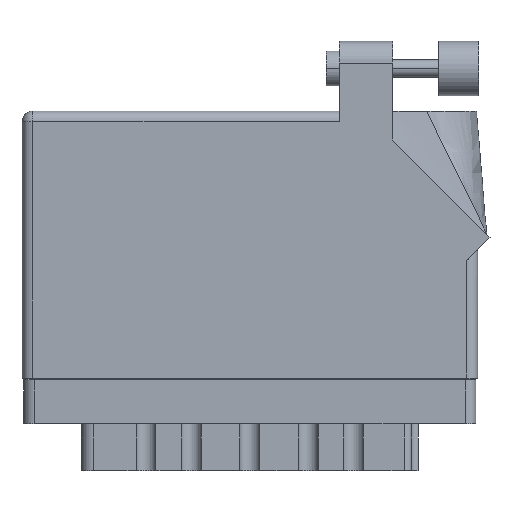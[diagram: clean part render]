
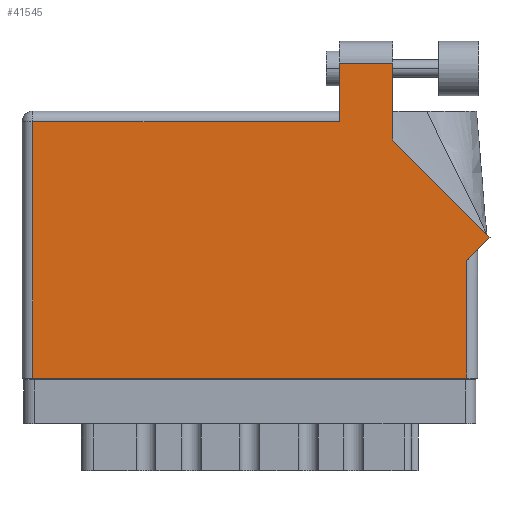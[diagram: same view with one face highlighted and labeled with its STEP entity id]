
A CAD part, front view. The second image highlights one B-rep face of the part: STEP entity #41545.
In plain terms, the highlighted face is planar.
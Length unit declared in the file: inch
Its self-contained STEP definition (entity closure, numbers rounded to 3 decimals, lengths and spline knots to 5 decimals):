
#160 = ORIENTED_EDGE ( 'NONE', *, *, #43689, .T. ) ;
#898 = CARTESIAN_POINT ( 'NONE',  ( 2.126, 1.36442, 0. ) ) ;
#1130 = VECTOR ( 'NONE', #20860, 39.37008 ) ;
#1275 = LINE ( 'NONE', #50636, #2593 ) ;
#1471 = VECTOR ( 'NONE', #4414, 39.37008 ) ;
#2537 = DIRECTION ( 'NONE',  ( -1., 0., 0. ) ) ;
#2593 = VECTOR ( 'NONE', #46176, 39.37008 ) ;
#2642 = CARTESIAN_POINT ( 'NONE',  ( 0., 1.53, 0. ) ) ;
#2730 = VERTEX_POINT ( 'NONE', #9732 ) ;
#2821 = CARTESIAN_POINT ( 'NONE',  ( 1.819, 1.805, 0. ) ) ;
#3860 = VECTOR ( 'NONE', #30760, 39.37008 ) ;
#4414 = DIRECTION ( 'NONE',  ( 0., -1., 0. ) ) ;
#6308 = CARTESIAN_POINT ( 'NONE',  ( 2.55, 0., 0. ) ) ;
#7575 = VERTEX_POINT ( 'NONE', #21977 ) ;
#7707 = VERTEX_POINT ( 'NONE', #2821 ) ;
#8414 = EDGE_CURVE ( 'NONE', #21898, #45044, #1275, .T. ) ;
#8733 = ORIENTED_EDGE ( 'NONE', *, *, #31412, .T. ) ;
#9506 = EDGE_CURVE ( 'NONE', #45044, #24134, #15478, .T. ) ;
#9732 = CARTESIAN_POINT ( 'NONE',  ( 2.126, 1.805, 0. ) ) ;
#10077 = CARTESIAN_POINT ( 'NONE',  ( 0.062, 0., 0. ) ) ;
#10794 = PLANE ( 'NONE',  #29612 ) ;
#10846 = VECTOR ( 'NONE', #25342, 39.37008 ) ;
#10869 = LINE ( 'NONE', #20679, #1130 ) ;
#12183 = ORIENTED_EDGE ( 'NONE', *, *, #40140, .T. ) ;
#12293 = CARTESIAN_POINT ( 'NONE',  ( 2.55, 0.675, 0. ) ) ;
#12740 = VERTEX_POINT ( 'NONE', #34656 ) ;
#13725 = VECTOR ( 'NONE', #2537, 39.37008 ) ;
#13726 = EDGE_CURVE ( 'NONE', #28199, #7575, #24743, .T. ) ;
#13822 = CARTESIAN_POINT ( 'NONE',  ( 2.68271, 0.80771, 0. ) ) ;
#14258 = DIRECTION ( 'NONE',  ( -1., 0., 0. ) ) ;
#14542 = CARTESIAN_POINT ( 'NONE',  ( 2.55, 0.737, 0. ) ) ;
#14940 = ORIENTED_EDGE ( 'NONE', *, *, #13726, .T. ) ;
#15335 = EDGE_CURVE ( 'NONE', #7575, #21898, #50003, .T. ) ;
#15451 = CARTESIAN_POINT ( 'NONE',  ( 2.612, 0.737, 0. ) ) ;
#15478 = LINE ( 'NONE', #14542, #3860 ) ;
#16830 = LINE ( 'NONE', #15451, #38223 ) ;
#16868 = ORIENTED_EDGE ( 'NONE', *, *, #9506, .T. ) ;
#17122 = ORIENTED_EDGE ( 'NONE', *, *, #26634, .T. ) ;
#20679 = CARTESIAN_POINT ( 'NONE',  ( 1.819, 1.53, 0. ) ) ;
#20794 = VECTOR ( 'NONE', #47097, 39.37008 ) ;
#20860 = DIRECTION ( 'NONE',  ( 0., -1., 0. ) ) ;
#21806 = LINE ( 'NONE', #898, #10846 ) ;
#21898 = VERTEX_POINT ( 'NONE', #10077 ) ;
#21977 = CARTESIAN_POINT ( 'NONE',  ( 0.062, 1.468, 0. ) ) ;
#22461 = EDGE_LOOP ( 'NONE', ( #12183, #17122, #52082, #14940, #33768, #53384, #16868, #8733, #160 ) ) ;
#24134 = VERTEX_POINT ( 'NONE', #12293 ) ;
#24701 = CARTESIAN_POINT ( 'NONE',  ( 0.062, 0., 0. ) ) ;
#24743 = LINE ( 'NONE', #44180, #13725 ) ;
#25342 = DIRECTION ( 'NONE',  ( 0., 1., 0. ) ) ;
#25583 = LINE ( 'NONE', #51855, #48249 ) ;
#26634 = EDGE_CURVE ( 'NONE', #2730, #7707, #25583, .T. ) ;
#27177 = DIRECTION ( 'NONE',  ( 0.707, 0.707, 0. ) ) ;
#28199 = VERTEX_POINT ( 'NONE', #52750 ) ;
#29612 = AXIS2_PLACEMENT_3D ( 'NONE', #2642, #31526, #47690 ) ;
#30461 = LINE ( 'NONE', #13822, #20794 ) ;
#30760 = DIRECTION ( 'NONE',  ( 0., 1., 0. ) ) ;
#31412 = EDGE_CURVE ( 'NONE', #24134, #47686, #16830, .T. ) ;
#31526 = DIRECTION ( 'NONE',  ( 0., 0., -1. ) ) ;
#33768 = ORIENTED_EDGE ( 'NONE', *, *, #15335, .T. ) ;
#34656 = CARTESIAN_POINT ( 'NONE',  ( 2.126, 1.36442, 0. ) ) ;
#37341 = FACE_OUTER_BOUND ( 'NONE', #22461, .T. ) ;
#38223 = VECTOR ( 'NONE', #27177, 39.37008 ) ;
#40140 = EDGE_CURVE ( 'NONE', #12740, #2730, #21806, .T. ) ;
#41545 = ADVANCED_FACE ( 'NONE', ( #37341 ), #10794, .F. ) ;
#43689 = EDGE_CURVE ( 'NONE', #47686, #12740, #30461, .T. ) ;
#44180 = CARTESIAN_POINT ( 'NONE',  ( 0., 1.468, 0. ) ) ;
#45044 = VERTEX_POINT ( 'NONE', #6308 ) ;
#46176 = DIRECTION ( 'NONE',  ( 1., 0., 0. ) ) ;
#47077 = EDGE_CURVE ( 'NONE', #7707, #28199, #10869, .T. ) ;
#47097 = DIRECTION ( 'NONE',  ( -0.707, 0.707, 0. ) ) ;
#47686 = VERTEX_POINT ( 'NONE', #48526 ) ;
#47690 = DIRECTION ( 'NONE',  ( -1., 0., 0. ) ) ;
#48249 = VECTOR ( 'NONE', #14258, 39.37008 ) ;
#48526 = CARTESIAN_POINT ( 'NONE',  ( 2.68271, 0.80771, 0. ) ) ;
#50003 = LINE ( 'NONE', #24701, #1471 ) ;
#50636 = CARTESIAN_POINT ( 'NONE',  ( 0., 0., 0. ) ) ;
#51855 = CARTESIAN_POINT ( 'NONE',  ( 1.819, 1.805, 0. ) ) ;
#52082 = ORIENTED_EDGE ( 'NONE', *, *, #47077, .T. ) ;
#52750 = CARTESIAN_POINT ( 'NONE',  ( 1.819, 1.468, 0. ) ) ;
#53384 = ORIENTED_EDGE ( 'NONE', *, *, #8414, .T. ) ;
